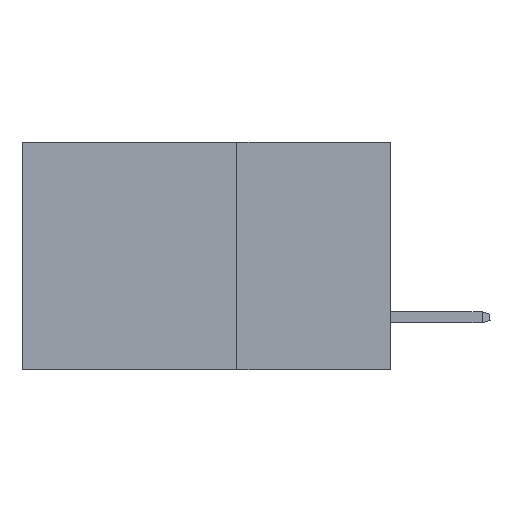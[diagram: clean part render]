
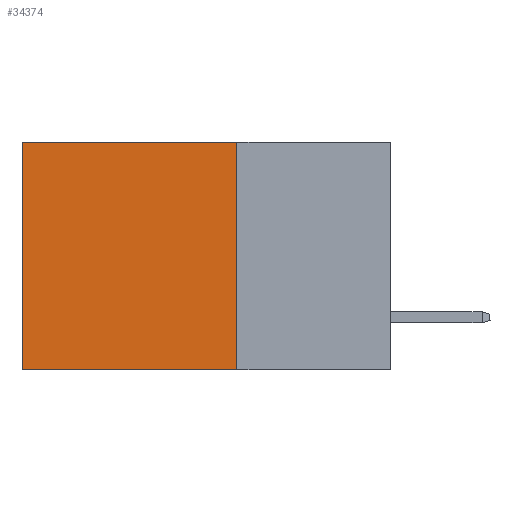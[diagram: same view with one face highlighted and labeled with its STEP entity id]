
A CAD part, left-side view. The second image highlights one B-rep face of the part: STEP entity #34374.
In plain terms, the highlighted planar face has unit normal (-1, 0, 0).
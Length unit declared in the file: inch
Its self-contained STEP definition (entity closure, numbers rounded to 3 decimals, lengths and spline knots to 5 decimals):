
#108 = ORIENTED_EDGE ( 'NONE', *, *, #36528, .T. ) ;
#654 = EDGE_LOOP ( 'NONE', ( #108, #35051, #5286, #7092 ) ) ;
#5286 = ORIENTED_EDGE ( 'NONE', *, *, #6178, .F. ) ;
#6178 = EDGE_CURVE ( 'NONE', #31774, #9892, #18254, .T. ) ;
#6359 = VECTOR ( 'NONE', #23883, 39.37008 ) ;
#7092 = ORIENTED_EDGE ( 'NONE', *, *, #31177, .T. ) ;
#8275 = CARTESIAN_POINT ( 'NONE',  ( 0.2875, 0.6, -0.37 ) ) ;
#8555 = CARTESIAN_POINT ( 'NONE',  ( 0.2875, 0.25, -0.37 ) ) ;
#8781 = DIRECTION ( 'NONE',  ( 0., 0., -1. ) ) ;
#9772 = FACE_OUTER_BOUND ( 'NONE', #654, .T. ) ;
#9892 = VERTEX_POINT ( 'NONE', #8555 ) ;
#10102 = VERTEX_POINT ( 'NONE', #35425 ) ;
#10867 = DIRECTION ( 'NONE',  ( 0., 1., 0. ) ) ;
#12594 = PLANE ( 'NONE',  #23617 ) ;
#13316 = CARTESIAN_POINT ( 'NONE',  ( 0.2875, 0.25, 0. ) ) ;
#16734 = LINE ( 'NONE', #37726, #6359 ) ;
#17820 = VECTOR ( 'NONE', #10867, 39.37008 ) ;
#18254 = LINE ( 'NONE', #38199, #35747 ) ;
#20527 = DIRECTION ( 'NONE',  ( 0., 0., -1. ) ) ;
#23029 = EDGE_CURVE ( 'NONE', #9892, #41651, #45116, .T. ) ;
#23617 = AXIS2_PLACEMENT_3D ( 'NONE', #37169, #43587, #8781 ) ;
#23883 = DIRECTION ( 'NONE',  ( 0., 0., -1. ) ) ;
#24591 = CARTESIAN_POINT ( 'NONE',  ( 0.2875, 0.25, 0. ) ) ;
#25105 = CARTESIAN_POINT ( 'NONE',  ( 0.2875, 0.25, -0.37 ) ) ;
#27603 = DIRECTION ( 'NONE',  ( 0., 1., 0. ) ) ;
#27752 = LINE ( 'NONE', #24591, #35939 ) ;
#31177 = EDGE_CURVE ( 'NONE', #31774, #10102, #27752, .T. ) ;
#31774 = VERTEX_POINT ( 'NONE', #13316 ) ;
#34374 = ADVANCED_FACE ( 'NONE', ( #9772 ), #12594, .F. ) ;
#35051 = ORIENTED_EDGE ( 'NONE', *, *, #23029, .F. ) ;
#35425 = CARTESIAN_POINT ( 'NONE',  ( 0.2875, 0.6, 0. ) ) ;
#35747 = VECTOR ( 'NONE', #20527, 39.37008 ) ;
#35939 = VECTOR ( 'NONE', #27603, 39.37008 ) ;
#36528 = EDGE_CURVE ( 'NONE', #10102, #41651, #16734, .T. ) ;
#37169 = CARTESIAN_POINT ( 'NONE',  ( 0.2875, 0.25, 0. ) ) ;
#37726 = CARTESIAN_POINT ( 'NONE',  ( 0.2875, 0.6, 0. ) ) ;
#38199 = CARTESIAN_POINT ( 'NONE',  ( 0.2875, 0.25, 0. ) ) ;
#41651 = VERTEX_POINT ( 'NONE', #8275 ) ;
#43587 = DIRECTION ( 'NONE',  ( 1., 0., 0. ) ) ;
#45116 = LINE ( 'NONE', #25105, #17820 ) ;
